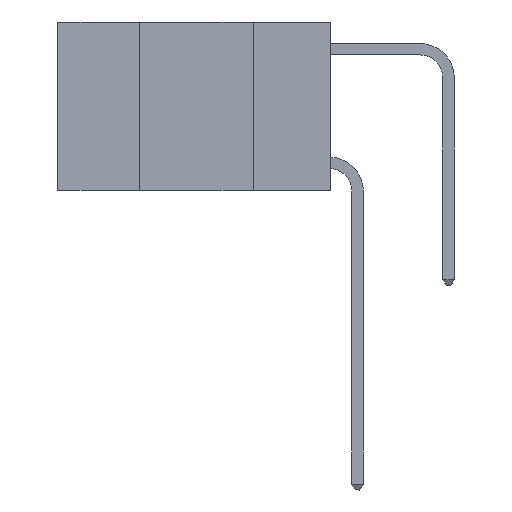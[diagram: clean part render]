
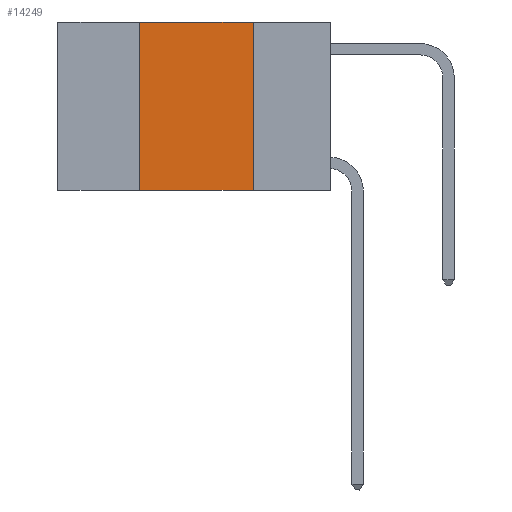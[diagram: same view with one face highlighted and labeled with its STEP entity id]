
A CAD part, left-side view. The second image highlights one B-rep face of the part: STEP entity #14249.
In plain terms, the highlighted planar face has unit normal (-1, 0, 0).
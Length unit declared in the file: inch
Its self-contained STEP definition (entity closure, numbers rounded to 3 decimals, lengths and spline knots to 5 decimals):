
#306 = CARTESIAN_POINT ( 'NONE',  ( 0., 0.6, 0. ) ) ;
#975 = DIRECTION ( 'NONE',  ( 0., -1., 0. ) ) ;
#1578 = FACE_OUTER_BOUND ( 'NONE', #10996, .T. ) ;
#1898 = ORIENTED_EDGE ( 'NONE', *, *, #5543, .T. ) ;
#2956 = EDGE_CURVE ( 'NONE', #7020, #13177, #14114, .T. ) ;
#3053 = EDGE_CURVE ( 'NONE', #10410, #13336, #12683, .T. ) ;
#3075 = VECTOR ( 'NONE', #9444, 39.37008 ) ;
#3765 = VECTOR ( 'NONE', #6204, 39.37008 ) ;
#3911 = ORIENTED_EDGE ( 'NONE', *, *, #2956, .F. ) ;
#5187 = EDGE_CURVE ( 'NONE', #13336, #7020, #9944, .T. ) ;
#5543 = EDGE_CURVE ( 'NONE', #10410, #13177, #11384, .T. ) ;
#6010 = VECTOR ( 'NONE', #975, 39.37008 ) ;
#6204 = DIRECTION ( 'NONE',  ( 0., -1., 0. ) ) ;
#6520 = DIRECTION ( 'NONE',  ( 0., 0., -1. ) ) ;
#6721 = CARTESIAN_POINT ( 'NONE',  ( 0., 0.42, 0. ) ) ;
#7020 = VERTEX_POINT ( 'NONE', #12742 ) ;
#7146 = CARTESIAN_POINT ( 'NONE',  ( 0., 0.42, 0. ) ) ;
#7600 = CARTESIAN_POINT ( 'NONE',  ( 0., 0.17, -0.37 ) ) ;
#8011 = CARTESIAN_POINT ( 'NONE',  ( 0., 0.6, -0.37 ) ) ;
#9215 = CARTESIAN_POINT ( 'NONE',  ( 0., 0.17, 0. ) ) ;
#9444 = DIRECTION ( 'NONE',  ( 0., 0., 1. ) ) ;
#9944 = LINE ( 'NONE', #306, #3765 ) ;
#10334 = CARTESIAN_POINT ( 'NONE',  ( 0., 0.42, -0.37 ) ) ;
#10410 = VERTEX_POINT ( 'NONE', #10334 ) ;
#10707 = VECTOR ( 'NONE', #14945, 39.37008 ) ;
#10806 = ORIENTED_EDGE ( 'NONE', *, *, #3053, .F. ) ;
#10996 = EDGE_LOOP ( 'NONE', ( #3911, #13496, #10806, #1898 ) ) ;
#11384 = LINE ( 'NONE', #8011, #6010 ) ;
#12045 = AXIS2_PLACEMENT_3D ( 'NONE', #13323, #13368, #6520 ) ;
#12219 = PLANE ( 'NONE',  #12045 ) ;
#12683 = LINE ( 'NONE', #7146, #3075 ) ;
#12742 = CARTESIAN_POINT ( 'NONE',  ( 0., 0.17, 0. ) ) ;
#13177 = VERTEX_POINT ( 'NONE', #7600 ) ;
#13323 = CARTESIAN_POINT ( 'NONE',  ( 0., 0.6, 0. ) ) ;
#13336 = VERTEX_POINT ( 'NONE', #6721 ) ;
#13368 = DIRECTION ( 'NONE',  ( 1., 0., 0. ) ) ;
#13496 = ORIENTED_EDGE ( 'NONE', *, *, #5187, .F. ) ;
#14114 = LINE ( 'NONE', #9215, #10707 ) ;
#14249 = ADVANCED_FACE ( 'NONE', ( #1578 ), #12219, .F. ) ;
#14945 = DIRECTION ( 'NONE',  ( 0., 0., -1. ) ) ;
